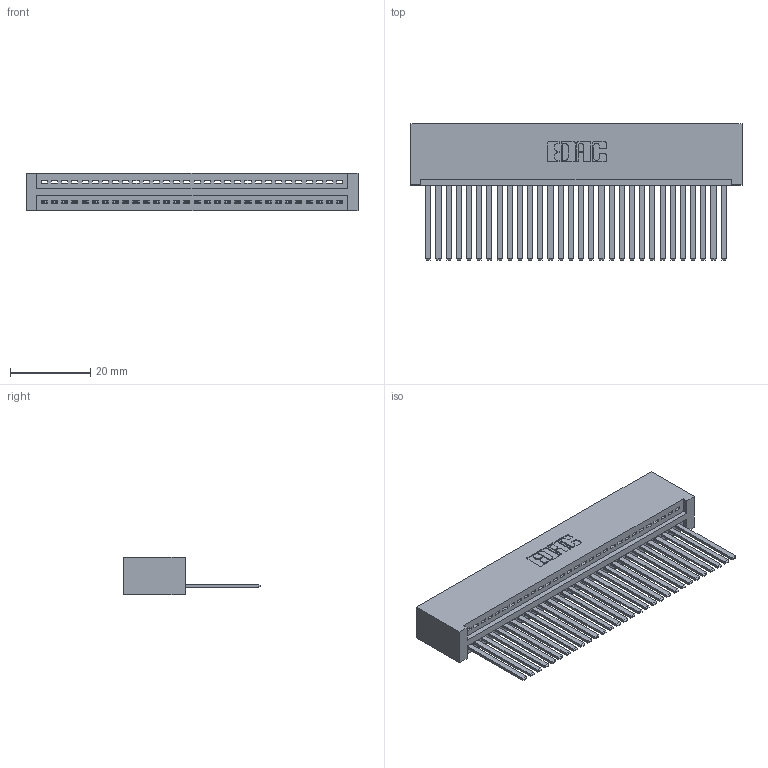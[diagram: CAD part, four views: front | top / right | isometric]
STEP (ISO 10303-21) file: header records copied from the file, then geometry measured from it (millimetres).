
FILE_DESCRIPTION (( 'STEP AP203' ), '1' );
FILE_NAME ('395-030-544-101.STEP', '2019-10-19T07:39:25', ( '' ), ( '' ), 'SwSTEP 2.0', 'SolidWorks 2016', '' );
FILE_SCHEMA (( 'CONFIG_CONTROL_DESIGN' ));
Length unit declared in the file: inch
Products named in the file (3): 345 Part_No Mounting Lugs; 345-292-001_345-293-144; 395-030-544-101
Assembly tree (31 placements, depth 2):
  395-030-544-101
    345 Part_No Mounting Lugs
    345-292-001_345-293-144  x30
Bounding box: 82.8 x 33.96 x 9.4 mm (x, y, z)
Volume: 8698.3 mm3; surface area: 12629.4 mm2
Topology: 31 solids, 31 shells, 1678 faces, 5057 edges, 3330 vertices
Faces by surface type: plane 1156, cylinder 522
Entity records: 23733 total; most frequent: CARTESIAN_POINT 4118, ORIENTED_EDGE 4082, DIRECTION 3605, EDGE_CURVE 2041, LINE 1801, VECTOR 1801, VERTEX_POINT 1358, AXIS2_PLACEMENT_3D 902
